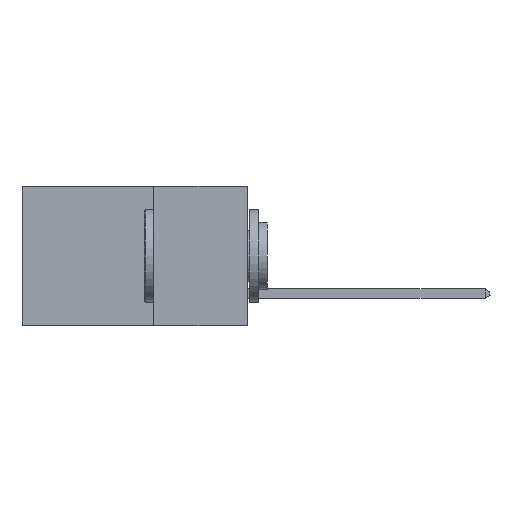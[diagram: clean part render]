
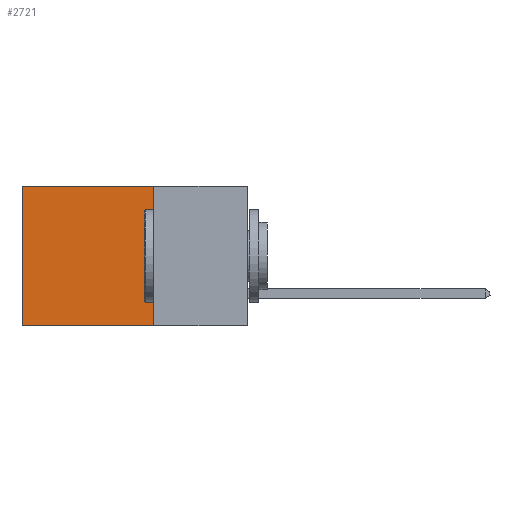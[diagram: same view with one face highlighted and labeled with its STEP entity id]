
A CAD part, left-side view. The second image highlights one B-rep face of the part: STEP entity #2721.
In plain terms, the highlighted planar face has unit normal (-1, 0, 0).
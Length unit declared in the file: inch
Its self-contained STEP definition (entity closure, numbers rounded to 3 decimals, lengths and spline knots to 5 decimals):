
#964 = ORIENTED_EDGE ( 'NONE', *, *, #9493, .T. ) ;
#1898 = CARTESIAN_POINT ( 'NONE',  ( 0.298, 0.25, -0.37 ) ) ;
#2721 = ADVANCED_FACE ( 'NONE', ( #13527 ), #8889, .F. ) ;
#3033 = CARTESIAN_POINT ( 'NONE',  ( 0.298, 0.25, 0. ) ) ;
#3996 = AXIS2_PLACEMENT_3D ( 'NONE', #22480, #13623, #4775 ) ;
#4037 = VECTOR ( 'NONE', #25355, 39.37008 ) ;
#4248 = ORIENTED_EDGE ( 'NONE', *, *, #21029, .T. ) ;
#4345 = EDGE_CURVE ( 'NONE', #24182, #23089, #11708, .T. ) ;
#4775 = DIRECTION ( 'NONE',  ( 0., 0., -1. ) ) ;
#5664 = CARTESIAN_POINT ( 'NONE',  ( 0.298, 0.25, 0. ) ) ;
#5827 = CARTESIAN_POINT ( 'NONE',  ( 0.298, 0.6, 0. ) ) ;
#7150 = CARTESIAN_POINT ( 'NONE',  ( 0.298, 0.25, -0.37 ) ) ;
#7264 = LINE ( 'NONE', #3033, #26022 ) ;
#8315 = DIRECTION ( 'NONE',  ( 0., 0., -1. ) ) ;
#8426 = CARTESIAN_POINT ( 'NONE',  ( 0.298, 0.6, 0. ) ) ;
#8574 = VECTOR ( 'NONE', #8315, 39.37008 ) ;
#8889 = PLANE ( 'NONE',  #3996 ) ;
#9493 = EDGE_CURVE ( 'NONE', #21742, #25653, #21093, .T. ) ;
#9749 = CARTESIAN_POINT ( 'NONE',  ( 0.298, 0.6, -0.37 ) ) ;
#9862 = ORIENTED_EDGE ( 'NONE', *, *, #11077, .F. ) ;
#11077 = EDGE_CURVE ( 'NONE', #23089, #25653, #15798, .T. ) ;
#11407 = EDGE_LOOP ( 'NONE', ( #964, #9862, #28285, #4248 ) ) ;
#11708 = LINE ( 'NONE', #12239, #4037 ) ;
#12239 = CARTESIAN_POINT ( 'NONE',  ( 0.298, 0.25, 0. ) ) ;
#12822 = DIRECTION ( 'NONE',  ( 0., 1., 0. ) ) ;
#13527 = FACE_OUTER_BOUND ( 'NONE', #11407, .T. ) ;
#13623 = DIRECTION ( 'NONE',  ( 1., 0., 0. ) ) ;
#15798 = LINE ( 'NONE', #1898, #24168 ) ;
#16270 = DIRECTION ( 'NONE',  ( 0., 1., 0. ) ) ;
#21029 = EDGE_CURVE ( 'NONE', #24182, #21742, #7264, .T. ) ;
#21093 = LINE ( 'NONE', #8426, #8574 ) ;
#21742 = VERTEX_POINT ( 'NONE', #5827 ) ;
#22480 = CARTESIAN_POINT ( 'NONE',  ( 0.298, 0.25, 0. ) ) ;
#23089 = VERTEX_POINT ( 'NONE', #7150 ) ;
#24168 = VECTOR ( 'NONE', #12822, 39.37008 ) ;
#24182 = VERTEX_POINT ( 'NONE', #5664 ) ;
#25355 = DIRECTION ( 'NONE',  ( 0., 0., -1. ) ) ;
#25653 = VERTEX_POINT ( 'NONE', #9749 ) ;
#26022 = VECTOR ( 'NONE', #16270, 39.37008 ) ;
#28285 = ORIENTED_EDGE ( 'NONE', *, *, #4345, .F. ) ;
